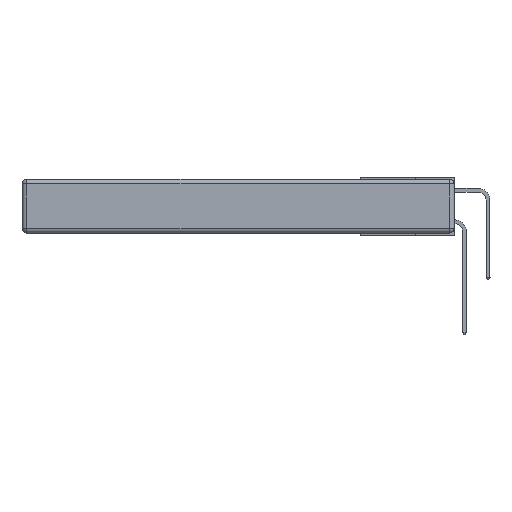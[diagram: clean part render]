
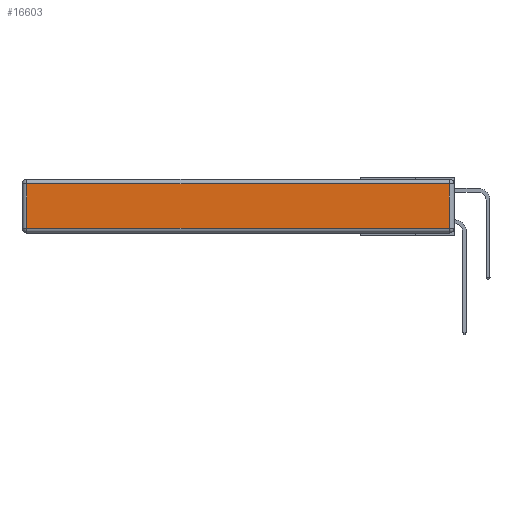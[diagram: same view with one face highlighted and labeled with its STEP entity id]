
A CAD part, left-side view. The second image highlights one B-rep face of the part: STEP entity #16603.
In plain terms, the highlighted planar face has unit normal (-1, 0, 0).
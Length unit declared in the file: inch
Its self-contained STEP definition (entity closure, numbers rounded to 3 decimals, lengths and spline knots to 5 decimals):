
#1907 = DIRECTION ( 'NONE',  ( 0., 0., 1. ) ) ;
#2053 = VECTOR ( 'NONE', #1907, 39.37008 ) ;
#2493 = AXIS2_PLACEMENT_3D ( 'NONE', #5979, #5793, #19892 ) ;
#5410 = EDGE_LOOP ( 'NONE', ( #18050, #8828, #7686, #22346 ) ) ;
#5510 = LINE ( 'NONE', #7237, #20954 ) ;
#5511 = VERTEX_POINT ( 'NONE', #16898 ) ;
#5793 = DIRECTION ( 'NONE',  ( -1., 0., 0. ) ) ;
#5979 = CARTESIAN_POINT ( 'NONE',  ( 0., 0., -0.343 ) ) ;
#7237 = CARTESIAN_POINT ( 'NONE',  ( 0., 2.75, -0.03 ) ) ;
#7686 = ORIENTED_EDGE ( 'NONE', *, *, #13633, .T. ) ;
#7788 = EDGE_CURVE ( 'NONE', #9873, #23016, #8918, .T. ) ;
#8828 = ORIENTED_EDGE ( 'NONE', *, *, #17168, .T. ) ;
#8918 = LINE ( 'NONE', #15213, #9558 ) ;
#9558 = VECTOR ( 'NONE', #17328, 39.37008 ) ;
#9646 = DIRECTION ( 'NONE',  ( 0., 0., -1. ) ) ;
#9873 = VERTEX_POINT ( 'NONE', #11277 ) ;
#10107 = PLANE ( 'NONE',  #2493 ) ;
#11277 = CARTESIAN_POINT ( 'NONE',  ( 0., 2.72, -0.313 ) ) ;
#12052 = CARTESIAN_POINT ( 'NONE',  ( 0., 0.03, -0.343 ) ) ;
#12680 = CARTESIAN_POINT ( 'NONE',  ( 0., 0.03, -0.313 ) ) ;
#13633 = EDGE_CURVE ( 'NONE', #23831, #5511, #5510, .T. ) ;
#15213 = CARTESIAN_POINT ( 'NONE',  ( 0., 0., -0.313 ) ) ;
#16603 = ADVANCED_FACE ( 'NONE', ( #19130 ), #10107, .T. ) ;
#16898 = CARTESIAN_POINT ( 'NONE',  ( 0., 2.72, -0.03 ) ) ;
#17168 = EDGE_CURVE ( 'NONE', #23016, #23831, #18780, .T. ) ;
#17328 = DIRECTION ( 'NONE',  ( 0., -1., 0. ) ) ;
#17839 = CARTESIAN_POINT ( 'NONE',  ( 0., 2.72, -0.343 ) ) ;
#18050 = ORIENTED_EDGE ( 'NONE', *, *, #7788, .T. ) ;
#18058 = DIRECTION ( 'NONE',  ( 0., 1., 0. ) ) ;
#18500 = LINE ( 'NONE', #17839, #25751 ) ;
#18780 = LINE ( 'NONE', #12052, #2053 ) ;
#19130 = FACE_OUTER_BOUND ( 'NONE', #5410, .T. ) ;
#19892 = DIRECTION ( 'NONE',  ( 0., 0., 1. ) ) ;
#20954 = VECTOR ( 'NONE', #18058, 39.37008 ) ;
#22346 = ORIENTED_EDGE ( 'NONE', *, *, #23813, .T. ) ;
#23016 = VERTEX_POINT ( 'NONE', #12680 ) ;
#23813 = EDGE_CURVE ( 'NONE', #5511, #9873, #18500, .T. ) ;
#23831 = VERTEX_POINT ( 'NONE', #25794 ) ;
#25751 = VECTOR ( 'NONE', #9646, 39.37008 ) ;
#25794 = CARTESIAN_POINT ( 'NONE',  ( 0., 0.03, -0.03 ) ) ;
